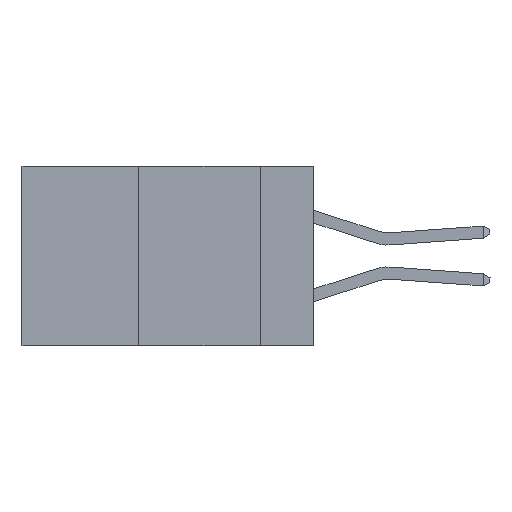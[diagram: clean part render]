
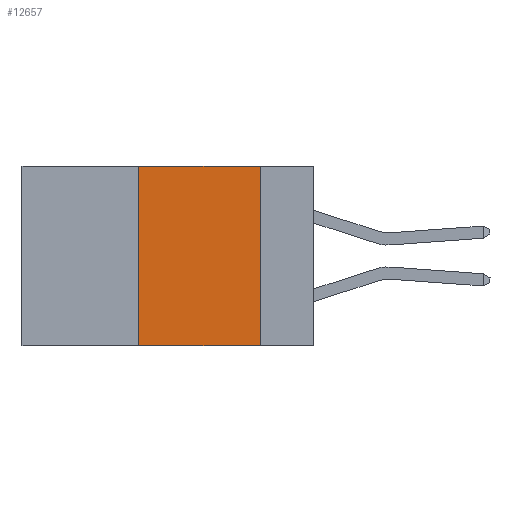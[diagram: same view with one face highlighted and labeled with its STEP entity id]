
A CAD part, left-side view. The second image highlights one B-rep face of the part: STEP entity #12657.
In plain terms, the highlighted planar face has unit normal (-1, 0, 0).
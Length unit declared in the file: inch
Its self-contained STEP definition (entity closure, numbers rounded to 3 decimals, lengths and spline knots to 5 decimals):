
#966 = LINE ( 'NONE', #7585, #8060 ) ;
#979 = LINE ( 'NONE', #15327, #7634 ) ;
#1367 = VERTEX_POINT ( 'NONE', #7894 ) ;
#1898 = LINE ( 'NONE', #2719, #15033 ) ;
#2023 = DIRECTION ( 'NONE',  ( 0., -1., 0. ) ) ;
#2719 = CARTESIAN_POINT ( 'NONE',  ( 0., 0.36, 0. ) ) ;
#2734 = EDGE_CURVE ( 'NONE', #9703, #12899, #1898, .T. ) ;
#2784 = LINE ( 'NONE', #16508, #17382 ) ;
#3096 = EDGE_CURVE ( 'NONE', #9703, #1367, #2784, .T. ) ;
#3136 = ORIENTED_EDGE ( 'NONE', *, *, #3096, .T. ) ;
#4403 = VERTEX_POINT ( 'NONE', #13799 ) ;
#4627 = ORIENTED_EDGE ( 'NONE', *, *, #13455, .F. ) ;
#4701 = EDGE_LOOP ( 'NONE', ( #4627, #16984, #7715, #3136 ) ) ;
#4756 = AXIS2_PLACEMENT_3D ( 'NONE', #7067, #8466, #17528 ) ;
#7067 = CARTESIAN_POINT ( 'NONE',  ( 0., 0.6, 0. ) ) ;
#7512 = EDGE_CURVE ( 'NONE', #12899, #4403, #966, .T. ) ;
#7585 = CARTESIAN_POINT ( 'NONE',  ( 0., 0.6, 0. ) ) ;
#7634 = VECTOR ( 'NONE', #16591, 39.37008 ) ;
#7715 = ORIENTED_EDGE ( 'NONE', *, *, #2734, .F. ) ;
#7894 = CARTESIAN_POINT ( 'NONE',  ( 0., 0.11, -0.37 ) ) ;
#8060 = VECTOR ( 'NONE', #2023, 39.37008 ) ;
#8466 = DIRECTION ( 'NONE',  ( 1., 0., 0. ) ) ;
#9703 = VERTEX_POINT ( 'NONE', #17506 ) ;
#10313 = CARTESIAN_POINT ( 'NONE',  ( 0., 0.36, 0. ) ) ;
#12657 = ADVANCED_FACE ( 'NONE', ( #13933 ), #15009, .F. ) ;
#12899 = VERTEX_POINT ( 'NONE', #10313 ) ;
#13455 = EDGE_CURVE ( 'NONE', #4403, #1367, #979, .T. ) ;
#13799 = CARTESIAN_POINT ( 'NONE',  ( 0., 0.11, 0. ) ) ;
#13933 = FACE_OUTER_BOUND ( 'NONE', #4701, .T. ) ;
#14881 = DIRECTION ( 'NONE',  ( 0., 0., 1. ) ) ;
#15009 = PLANE ( 'NONE',  #4756 ) ;
#15033 = VECTOR ( 'NONE', #14881, 39.37008 ) ;
#15327 = CARTESIAN_POINT ( 'NONE',  ( 0., 0.11, 0. ) ) ;
#16508 = CARTESIAN_POINT ( 'NONE',  ( 0., 0.6, -0.37 ) ) ;
#16591 = DIRECTION ( 'NONE',  ( 0., 0., -1. ) ) ;
#16705 = DIRECTION ( 'NONE',  ( 0., -1., 0. ) ) ;
#16984 = ORIENTED_EDGE ( 'NONE', *, *, #7512, .F. ) ;
#17382 = VECTOR ( 'NONE', #16705, 39.37008 ) ;
#17506 = CARTESIAN_POINT ( 'NONE',  ( 0., 0.36, -0.37 ) ) ;
#17528 = DIRECTION ( 'NONE',  ( 0., 0., -1. ) ) ;
